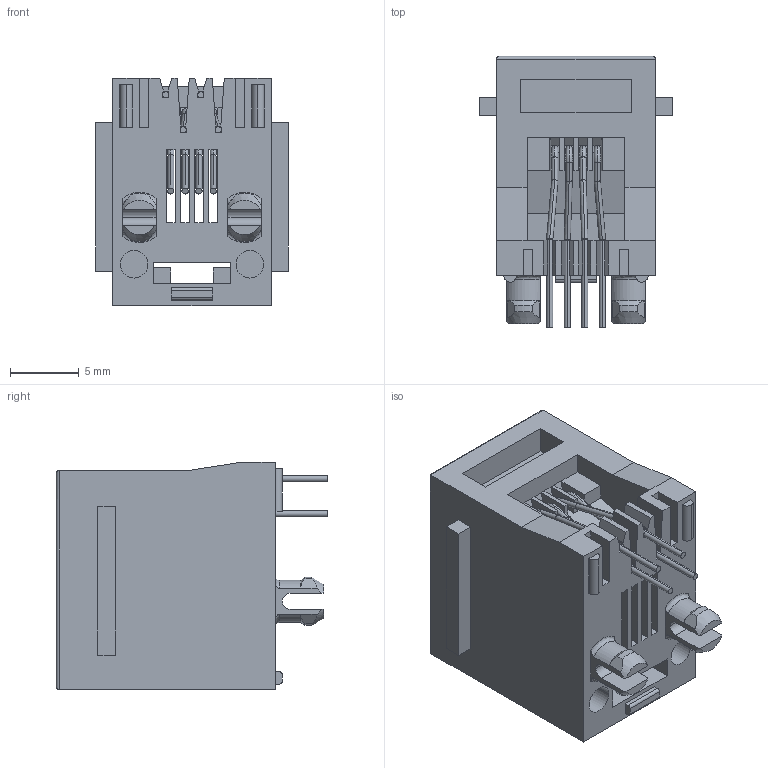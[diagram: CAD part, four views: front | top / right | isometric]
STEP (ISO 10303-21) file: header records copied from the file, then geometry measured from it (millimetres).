
FILE_DESCRIPTION (( 'STEP AP203' ), '1' );
FILE_NAME ('RJ21014491P00033.STEP', '2019-12-27T19:49:02', ( '' ), ( '' ), 'SwSTEP 2.0', 'SolidWorks 2016', '' );
FILE_SCHEMA (( 'CONFIG_CONTROL_DESIGN' ));
Length unit declared in the file: millimetre
Products named in the file (3): 21 Contacts; RJ21014491P00033; 21 Insulator
Assembly tree (2 placements, depth 2):
  RJ21014491P00033
    21 Insulator
    21 Contacts
Bounding box: 13.97 x 19.68 x 16.48 mm (x, y, z)
Volume: 1616.3 mm3; surface area: 2563.9 mm2
Topology: 5 solids, 5 shells, 369 faces, 969 edges, 608 vertices
Faces by surface type: plane 230, cylinder 111, torus 16, cone 8, bspline 4
Entity records: 11690 total; most frequent: CARTESIAN_POINT 2383, ORIENTED_EDGE 1938, DIRECTION 1801, EDGE_CURVE 969, LINE 709, VECTOR 709, VERTEX_POINT 608, AXIS2_PLACEMENT_3D 546
